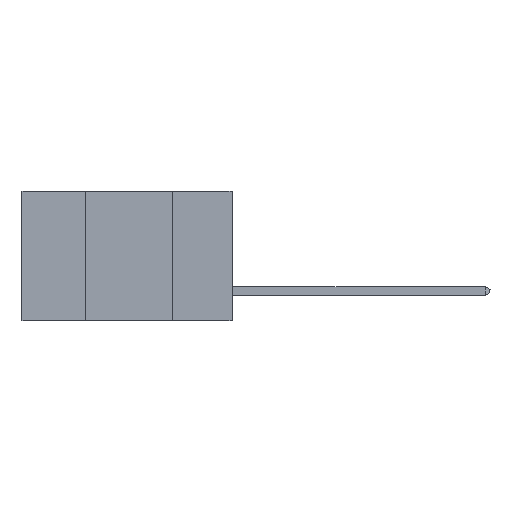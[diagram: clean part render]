
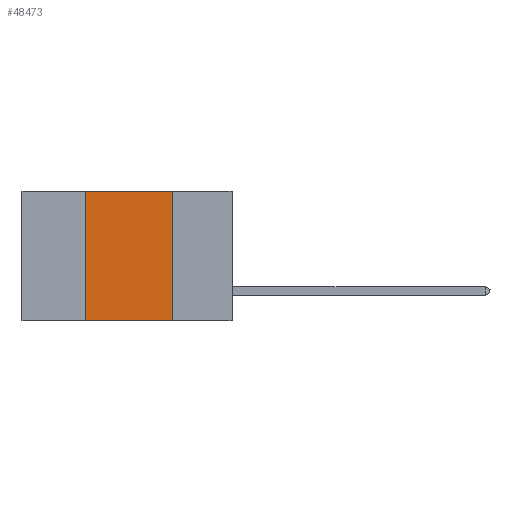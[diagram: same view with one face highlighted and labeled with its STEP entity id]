
A CAD part, left-side view. The second image highlights one B-rep face of the part: STEP entity #48473.
In plain terms, the highlighted planar face has unit normal (-1, 0, 0).
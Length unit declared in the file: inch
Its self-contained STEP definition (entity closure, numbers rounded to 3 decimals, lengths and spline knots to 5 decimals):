
#381 = CARTESIAN_POINT ( 'NONE',  ( 0., 0.6, 0. ) ) ;
#879 = CARTESIAN_POINT ( 'NONE',  ( 0., 0.17, -0.37 ) ) ;
#7898 = DIRECTION ( 'NONE',  ( 0., -1., 0. ) ) ;
#10159 = ORIENTED_EDGE ( 'NONE', *, *, #17330, .F. ) ;
#10358 = CARTESIAN_POINT ( 'NONE',  ( 0., 0.17, 0. ) ) ;
#10604 = CARTESIAN_POINT ( 'NONE',  ( 0., 0.17, 0. ) ) ;
#12391 = CARTESIAN_POINT ( 'NONE',  ( 0., 0.6, 0. ) ) ;
#13590 = LINE ( 'NONE', #45192, #36549 ) ;
#13952 = EDGE_CURVE ( 'NONE', #17240, #21002, #32865, .T. ) ;
#15004 = LINE ( 'NONE', #28737, #43282 ) ;
#17240 = VERTEX_POINT ( 'NONE', #21633 ) ;
#17330 = EDGE_CURVE ( 'NONE', #21002, #45933, #29117, .T. ) ;
#21002 = VERTEX_POINT ( 'NONE', #10358 ) ;
#21633 = CARTESIAN_POINT ( 'NONE',  ( 0., 0.42, 0. ) ) ;
#22558 = DIRECTION ( 'NONE',  ( 0., -1., 0. ) ) ;
#23005 = EDGE_CURVE ( 'NONE', #33447, #45933, #13590, .T. ) ;
#28737 = CARTESIAN_POINT ( 'NONE',  ( 0., 0.42, 0. ) ) ;
#29117 = LINE ( 'NONE', #10604, #45686 ) ;
#29539 = EDGE_LOOP ( 'NONE', ( #10159, #46473, #31341, #42588 ) ) ;
#30577 = DIRECTION ( 'NONE',  ( 1., 0., 0. ) ) ;
#30799 = AXIS2_PLACEMENT_3D ( 'NONE', #381, #30577, #34523 ) ;
#31341 = ORIENTED_EDGE ( 'NONE', *, *, #47226, .F. ) ;
#32185 = DIRECTION ( 'NONE',  ( 0., 0., 1. ) ) ;
#32865 = LINE ( 'NONE', #12391, #39415 ) ;
#33447 = VERTEX_POINT ( 'NONE', #42179 ) ;
#34523 = DIRECTION ( 'NONE',  ( 0., 0., -1. ) ) ;
#36549 = VECTOR ( 'NONE', #22558, 39.37008 ) ;
#37473 = DIRECTION ( 'NONE',  ( 0., 0., -1. ) ) ;
#39415 = VECTOR ( 'NONE', #7898, 39.37008 ) ;
#42165 = PLANE ( 'NONE',  #30799 ) ;
#42179 = CARTESIAN_POINT ( 'NONE',  ( 0., 0.42, -0.37 ) ) ;
#42588 = ORIENTED_EDGE ( 'NONE', *, *, #23005, .T. ) ;
#43282 = VECTOR ( 'NONE', #32185, 39.37008 ) ;
#45192 = CARTESIAN_POINT ( 'NONE',  ( 0., 0.6, -0.37 ) ) ;
#45686 = VECTOR ( 'NONE', #37473, 39.37008 ) ;
#45933 = VERTEX_POINT ( 'NONE', #879 ) ;
#46134 = FACE_OUTER_BOUND ( 'NONE', #29539, .T. ) ;
#46473 = ORIENTED_EDGE ( 'NONE', *, *, #13952, .F. ) ;
#47226 = EDGE_CURVE ( 'NONE', #33447, #17240, #15004, .T. ) ;
#48473 = ADVANCED_FACE ( 'NONE', ( #46134 ), #42165, .F. ) ;
